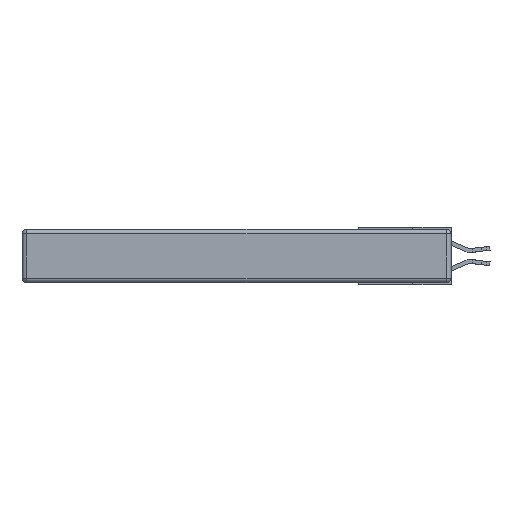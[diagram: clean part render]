
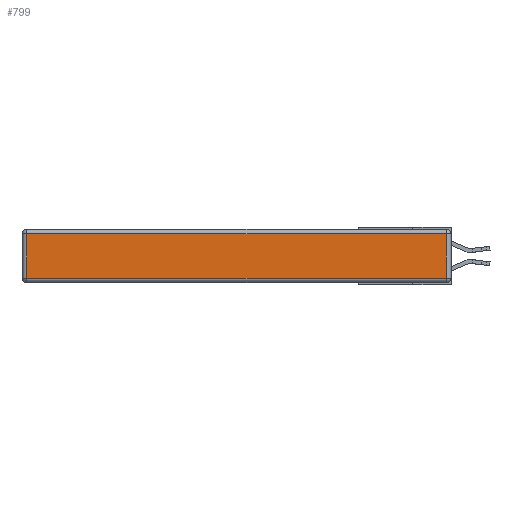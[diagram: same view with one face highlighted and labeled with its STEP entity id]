
A CAD part, left-side view. The second image highlights one B-rep face of the part: STEP entity #799.
In plain terms, the highlighted planar face has unit normal (-1, 0, 0).
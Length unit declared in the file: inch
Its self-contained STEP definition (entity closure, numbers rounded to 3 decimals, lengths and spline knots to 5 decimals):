
#186 = CARTESIAN_POINT ( 'NONE',  ( 0., 0., -0.313 ) ) ;
#518 = PLANE ( 'NONE',  #2153 ) ;
#519 = VECTOR ( 'NONE', #1220, 39.37008 ) ;
#575 = DIRECTION ( 'NONE',  ( 0., 0., 1. ) ) ;
#709 = CARTESIAN_POINT ( 'NONE',  ( 0., 2.72, -0.343 ) ) ;
#799 = ADVANCED_FACE ( 'NONE', ( #6552 ), #518, .T. ) ;
#1220 = DIRECTION ( 'NONE',  ( 0., 0., 1. ) ) ;
#2153 = AXIS2_PLACEMENT_3D ( 'NONE', #14405, #6847, #575 ) ;
#2464 = EDGE_LOOP ( 'NONE', ( #3832, #7481, #8490, #13003 ) ) ;
#3050 = EDGE_CURVE ( 'NONE', #12833, #7652, #13618, .T. ) ;
#3832 = ORIENTED_EDGE ( 'NONE', *, *, #14157, .T. ) ;
#4158 = VERTEX_POINT ( 'NONE', #11504 ) ;
#4435 = CARTESIAN_POINT ( 'NONE',  ( 0., 2.72, -0.03 ) ) ;
#4452 = CARTESIAN_POINT ( 'NONE',  ( 0., 0.03, -0.03 ) ) ;
#5063 = CARTESIAN_POINT ( 'NONE',  ( 0., 0.03, -0.343 ) ) ;
#6552 = FACE_OUTER_BOUND ( 'NONE', #2464, .T. ) ;
#6569 = VERTEX_POINT ( 'NONE', #6591 ) ;
#6591 = CARTESIAN_POINT ( 'NONE',  ( 0., 0.03, -0.313 ) ) ;
#6847 = DIRECTION ( 'NONE',  ( -1., 0., 0. ) ) ;
#6870 = DIRECTION ( 'NONE',  ( 0., 0., -1. ) ) ;
#7481 = ORIENTED_EDGE ( 'NONE', *, *, #7817, .T. ) ;
#7652 = VERTEX_POINT ( 'NONE', #4435 ) ;
#7817 = EDGE_CURVE ( 'NONE', #6569, #12833, #13944, .T. ) ;
#8490 = ORIENTED_EDGE ( 'NONE', *, *, #3050, .T. ) ;
#9111 = DIRECTION ( 'NONE',  ( 0., -1., 0. ) ) ;
#10988 = VECTOR ( 'NONE', #6870, 39.37008 ) ;
#11110 = EDGE_CURVE ( 'NONE', #7652, #4158, #15670, .T. ) ;
#11504 = CARTESIAN_POINT ( 'NONE',  ( 0., 2.72, -0.313 ) ) ;
#12833 = VERTEX_POINT ( 'NONE', #4452 ) ;
#13003 = ORIENTED_EDGE ( 'NONE', *, *, #11110, .T. ) ;
#13618 = LINE ( 'NONE', #14906, #14789 ) ;
#13844 = LINE ( 'NONE', #186, #15968 ) ;
#13944 = LINE ( 'NONE', #5063, #519 ) ;
#14157 = EDGE_CURVE ( 'NONE', #4158, #6569, #13844, .T. ) ;
#14405 = CARTESIAN_POINT ( 'NONE',  ( 0., 0., -0.343 ) ) ;
#14789 = VECTOR ( 'NONE', #14963, 39.37008 ) ;
#14906 = CARTESIAN_POINT ( 'NONE',  ( 0., 2.75, -0.03 ) ) ;
#14963 = DIRECTION ( 'NONE',  ( 0., 1., 0. ) ) ;
#15670 = LINE ( 'NONE', #709, #10988 ) ;
#15968 = VECTOR ( 'NONE', #9111, 39.37008 ) ;
